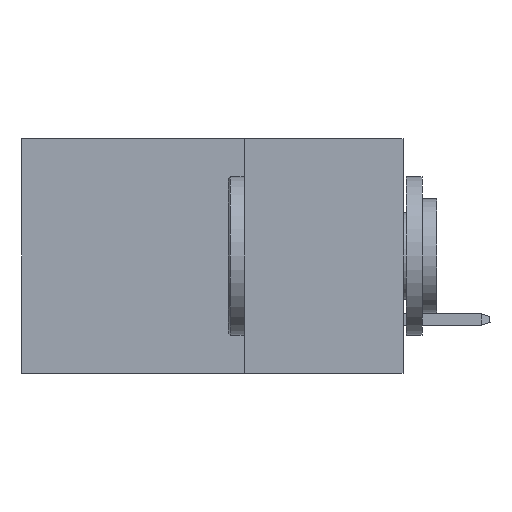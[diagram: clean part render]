
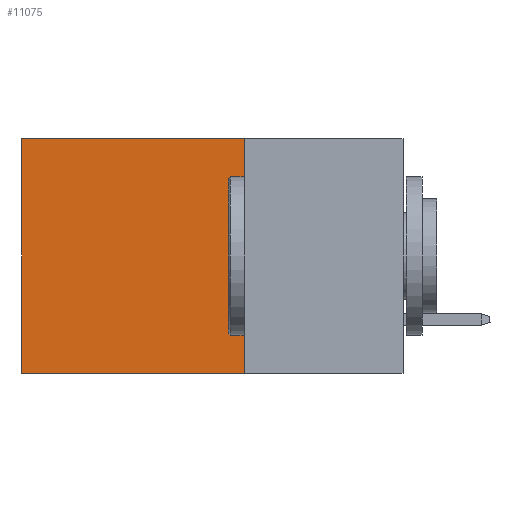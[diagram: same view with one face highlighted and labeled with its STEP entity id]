
A CAD part, left-side view. The second image highlights one B-rep face of the part: STEP entity #11075.
In plain terms, the highlighted planar face has unit normal (-1, 0, 0).
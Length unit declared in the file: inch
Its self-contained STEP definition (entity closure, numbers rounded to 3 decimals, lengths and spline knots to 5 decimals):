
#83 = DIRECTION ( 'NONE',  ( 0., 0., -1. ) ) ;
#266 = LINE ( 'NONE', #7190, #7761 ) ;
#1176 = EDGE_CURVE ( 'NONE', #16749, #5463, #10275, .T. ) ;
#1588 = EDGE_CURVE ( 'NONE', #5463, #9564, #266, .T. ) ;
#2523 = DIRECTION ( 'NONE',  ( 0., 1., 0. ) ) ;
#2808 = ORIENTED_EDGE ( 'NONE', *, *, #14202, .F. ) ;
#3089 = CARTESIAN_POINT ( 'NONE',  ( 0.2875, 0.25, 0. ) ) ;
#3261 = CARTESIAN_POINT ( 'NONE',  ( 0.2875, 0.25, 0. ) ) ;
#3439 = VERTEX_POINT ( 'NONE', #14807 ) ;
#5045 = VECTOR ( 'NONE', #9656, 39.37008 ) ;
#5463 = VERTEX_POINT ( 'NONE', #10766 ) ;
#5488 = EDGE_LOOP ( 'NONE', ( #7402, #7051, #2808, #9832 ) ) ;
#5826 = FACE_OUTER_BOUND ( 'NONE', #5488, .T. ) ;
#5907 = CARTESIAN_POINT ( 'NONE',  ( 0.2875, 0.25, 0. ) ) ;
#6103 = EDGE_CURVE ( 'NONE', #3439, #9564, #16487, .T. ) ;
#6772 = LINE ( 'NONE', #11006, #8484 ) ;
#7051 = ORIENTED_EDGE ( 'NONE', *, *, #6103, .F. ) ;
#7190 = CARTESIAN_POINT ( 'NONE',  ( 0.2875, 0.6, 0. ) ) ;
#7402 = ORIENTED_EDGE ( 'NONE', *, *, #1588, .T. ) ;
#7761 = VECTOR ( 'NONE', #83, 39.37008 ) ;
#8484 = VECTOR ( 'NONE', #9827, 39.37008 ) ;
#9564 = VERTEX_POINT ( 'NONE', #16281 ) ;
#9640 = CARTESIAN_POINT ( 'NONE',  ( 0.2875, 0.25, -0.37 ) ) ;
#9656 = DIRECTION ( 'NONE',  ( 0., 1., 0. ) ) ;
#9827 = DIRECTION ( 'NONE',  ( 0., 0., -1. ) ) ;
#9832 = ORIENTED_EDGE ( 'NONE', *, *, #1176, .T. ) ;
#10275 = LINE ( 'NONE', #5907, #5045 ) ;
#10326 = VECTOR ( 'NONE', #2523, 39.37008 ) ;
#10766 = CARTESIAN_POINT ( 'NONE',  ( 0.2875, 0.6, 0. ) ) ;
#11006 = CARTESIAN_POINT ( 'NONE',  ( 0.2875, 0.25, 0. ) ) ;
#11039 = AXIS2_PLACEMENT_3D ( 'NONE', #3261, #17045, #11568 ) ;
#11075 = ADVANCED_FACE ( 'NONE', ( #5826 ), #11473, .F. ) ;
#11473 = PLANE ( 'NONE',  #11039 ) ;
#11568 = DIRECTION ( 'NONE',  ( 0., 0., -1. ) ) ;
#14202 = EDGE_CURVE ( 'NONE', #16749, #3439, #6772, .T. ) ;
#14807 = CARTESIAN_POINT ( 'NONE',  ( 0.2875, 0.25, -0.37 ) ) ;
#16281 = CARTESIAN_POINT ( 'NONE',  ( 0.2875, 0.6, -0.37 ) ) ;
#16487 = LINE ( 'NONE', #9640, #10326 ) ;
#16749 = VERTEX_POINT ( 'NONE', #3089 ) ;
#17045 = DIRECTION ( 'NONE',  ( 1., 0., 0. ) ) ;
